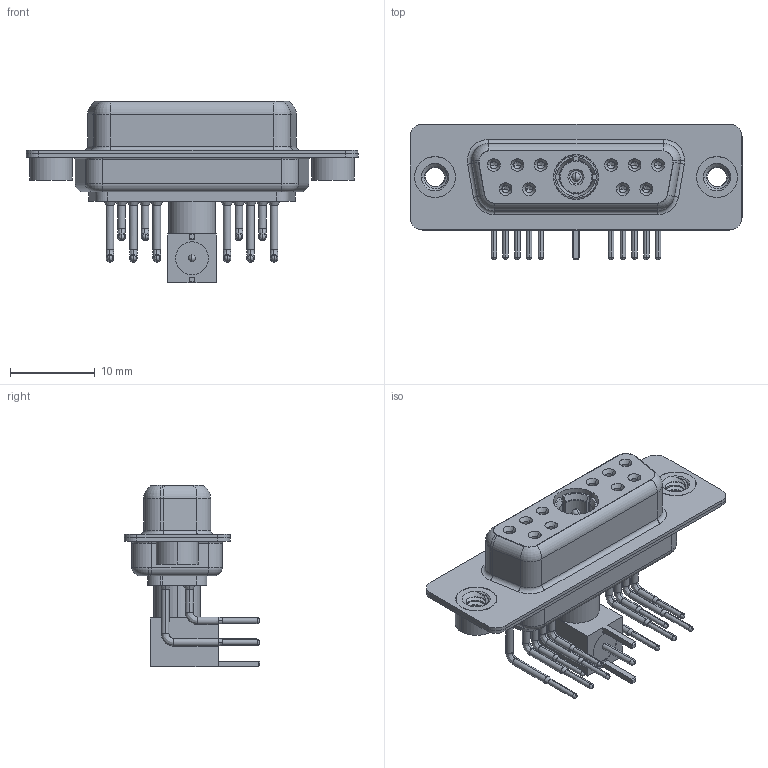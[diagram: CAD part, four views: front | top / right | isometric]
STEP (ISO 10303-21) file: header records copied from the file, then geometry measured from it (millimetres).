
FILE_DESCRIPTION (( 'STEP AP203' ), '1' );
FILE_NAME ('630-11W1240-7N2.STEP', '2022-05-31T09:58:40', ( '' ), ( '' ), 'SwSTEP 2.0', 'SolidWorks 2020', '' );
FILE_SCHEMA (( 'CONFIG_CONTROL_DESIGN' ));
Length unit declared in the file: millimetre
Products named in the file (14): 630-11W1240-7N2; Locking Collar; Co-Ax Plug_RA PC Tail; RA Back Shell; Pin_RA; 630Combo Shell Rear_15 Contacts; Insulator RA Pin; 630Combo Shell Front_15 Contacts; Insulator Pin_Straight PC Tail; Co-Ax Plug Assy_RA; 630Combo Threaded Rivet_2; 630Combo Housing_11W1; 630Combo Contact Row 2; 630Combo Contact Row 1
Assembly tree (22 placements, depth 3):
  630-11W1240-7N2
    630Combo Housing_11W1
    630Combo Shell Front_15 Contacts
    630Combo Shell Rear_15 Contacts
    630Combo Threaded Rivet_2  x2
    Co-Ax Plug Assy_RA
      Co-Ax Plug_RA PC Tail
      Insulator Pin_Straight PC Tail
      Pin_RA
      Locking Collar
      RA Back Shell
      Insulator RA Pin
    630Combo Contact Row 1  x6
    630Combo Contact Row 2  x4
Bounding box: 39.2 x 16 x 21.41 mm (x, y, z)
Volume: 2812.7 mm3; surface area: 6893.7 mm2
Topology: 21 solids, 21 shells, 977 faces, 2436 edges, 1528 vertices
Faces by surface type: cylinder 432, plane 284, cone 147, torus 63, bspline 47, sphere 4
Entity records: 21779 total; most frequent: CARTESIAN_POINT 5135, DIRECTION 3378, ORIENTED_EDGE 2958, EDGE_CURVE 1479, AXIS2_PLACEMENT_3D 1380, VERTEX_POINT 938, CIRCLE 742, EDGE_LOOP 727
